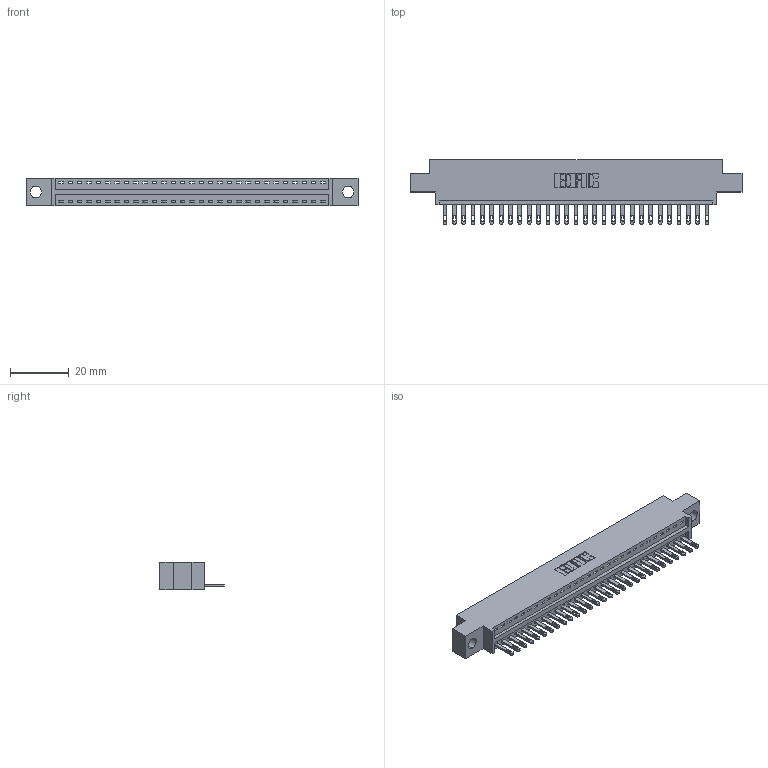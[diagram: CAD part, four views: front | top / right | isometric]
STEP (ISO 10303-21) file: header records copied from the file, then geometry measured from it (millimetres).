
FILE_DESCRIPTION (( 'STEP AP203' ), '1' );
FILE_NAME ('346-029-500-604.STEP', '2022-05-06T08:14:31', ( '' ), ( '' ), 'SwSTEP 2.0', 'SolidWorks 2020', '' );
FILE_SCHEMA (( 'CONFIG_CONTROL_DESIGN' ));
Length unit declared in the file: inch
Products named in the file (3): 345-292-001_345-293-100; 346-029-500-604; 346 Part_0.170 Offset - 0.156 Dia-TH
Assembly tree (30 placements, depth 2):
  346-029-500-604
    346 Part_0.170 Offset - 0.156 Dia-TH
    345-292-001_345-293-100  x29
Bounding box: 112.65 x 21.84 x 9.4 mm (x, y, z)
Volume: 10450.8 mm3; surface area: 12987.1 mm2
Topology: 30 solids, 30 shells, 1706 faces, 5249 edges, 3498 vertices
Faces by surface type: plane 1080, cylinder 626
Entity records: 20229 total; most frequent: CARTESIAN_POINT 3481, ORIENTED_EDGE 3442, DIRECTION 3087, EDGE_CURVE 1721, LINE 1469, VECTOR 1469, VERTEX_POINT 1146, AXIS2_PLACEMENT_3D 809
